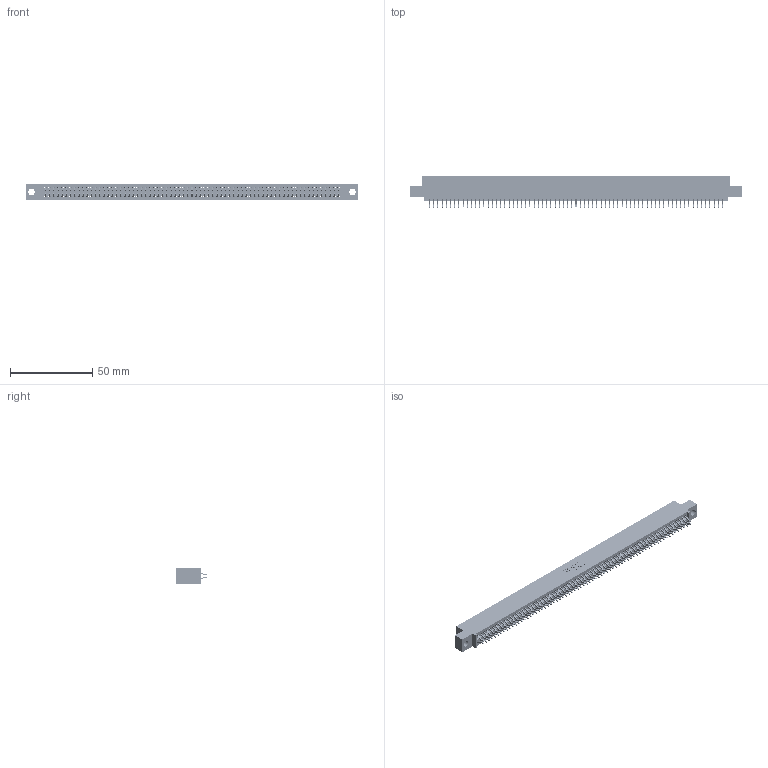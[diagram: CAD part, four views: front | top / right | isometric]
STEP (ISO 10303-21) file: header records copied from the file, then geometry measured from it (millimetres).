
FILE_DESCRIPTION (( 'STEP AP203' ), '1' );
FILE_NAME ('395-142-556-504.STEP', '2021-06-18T05:41:31', ( '' ), ( '' ), 'SwSTEP 2.0', 'SolidWorks 2020', '' );
FILE_SCHEMA (( 'CONFIG_CONTROL_DESIGN' ));
Length unit declared in the file: inch
Products named in the file (3): 345 Part_0.110 Offset - 0.156 Dia-TI; 345-292-001_556 Tail; 395-142-556-504
Assembly tree (143 placements, depth 2):
  395-142-556-504
    345 Part_0.110 Offset - 0.156 Dia-TI
    345-292-001_556 Tail  x142
Bounding box: 201.55 x 19.24 x 9.4 mm (x, y, z)
Volume: 19662.9 mm3; surface area: 29446.9 mm2
Topology: 143 solids, 143 shells, 8096 faces, 24103 edges, 15878 vertices
Faces by surface type: plane 5352, cylinder 2744
Entity records: 52575 total; most frequent: CARTESIAN_POINT 8806, ORIENTED_EDGE 8726, DIRECTION 7715, EDGE_CURVE 4363, LINE 3939, VECTOR 3939, VERTEX_POINT 2906, AXIS2_PLACEMENT_3D 1888
